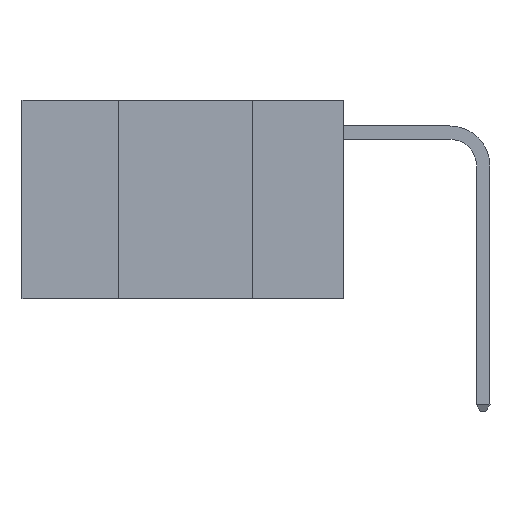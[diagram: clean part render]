
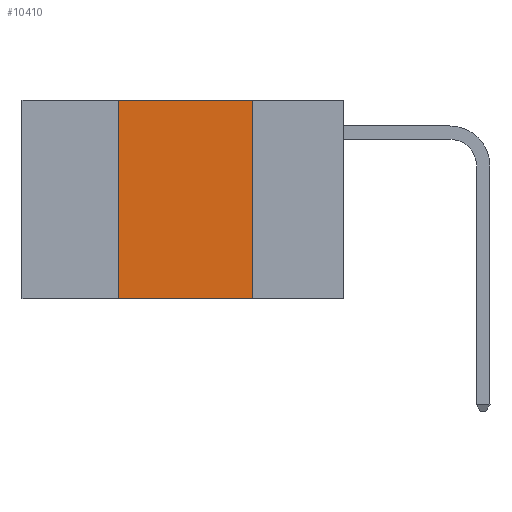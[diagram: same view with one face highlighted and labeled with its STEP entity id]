
A CAD part, left-side view. The second image highlights one B-rep face of the part: STEP entity #10410.
In plain terms, the highlighted planar face has unit normal (-1, 0, 0).
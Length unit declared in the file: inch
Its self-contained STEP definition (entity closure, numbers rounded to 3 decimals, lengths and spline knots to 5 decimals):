
#148 = PLANE ( 'NONE',  #8268 ) ;
#742 = CARTESIAN_POINT ( 'NONE',  ( 0., 0.6, -0.37 ) ) ;
#883 = EDGE_LOOP ( 'NONE', ( #10548, #9997, #11428, #1751 ) ) ;
#1121 = VERTEX_POINT ( 'NONE', #14163 ) ;
#1314 = DIRECTION ( 'NONE',  ( 0., 0., -1. ) ) ;
#1743 = LINE ( 'NONE', #13367, #4738 ) ;
#1751 = ORIENTED_EDGE ( 'NONE', *, *, #13897, .T. ) ;
#2292 = CARTESIAN_POINT ( 'NONE',  ( 0., 0.17, 0. ) ) ;
#2367 = DIRECTION ( 'NONE',  ( 0., 0., -1. ) ) ;
#2444 = VECTOR ( 'NONE', #2367, 39.37008 ) ;
#2475 = LINE ( 'NONE', #2292, #2444 ) ;
#2565 = EDGE_CURVE ( 'NONE', #1121, #4885, #2475, .T. ) ;
#3394 = EDGE_CURVE ( 'NONE', #5952, #9579, #13083, .T. ) ;
#4494 = LINE ( 'NONE', #742, #10064 ) ;
#4738 = VECTOR ( 'NONE', #6932, 39.37008 ) ;
#4885 = VERTEX_POINT ( 'NONE', #10338 ) ;
#5952 = VERTEX_POINT ( 'NONE', #7999 ) ;
#6932 = DIRECTION ( 'NONE',  ( 0., -1., 0. ) ) ;
#7334 = FACE_OUTER_BOUND ( 'NONE', #883, .T. ) ;
#7999 = CARTESIAN_POINT ( 'NONE',  ( 0., 0.42, -0.37 ) ) ;
#8111 = DIRECTION ( 'NONE',  ( 1., 0., 0. ) ) ;
#8268 = AXIS2_PLACEMENT_3D ( 'NONE', #10207, #8111, #1314 ) ;
#9579 = VERTEX_POINT ( 'NONE', #12835 ) ;
#9997 = ORIENTED_EDGE ( 'NONE', *, *, #12169, .F. ) ;
#10064 = VECTOR ( 'NONE', #11868, 39.37008 ) ;
#10207 = CARTESIAN_POINT ( 'NONE',  ( 0., 0.6, 0. ) ) ;
#10338 = CARTESIAN_POINT ( 'NONE',  ( 0., 0.17, -0.37 ) ) ;
#10410 = ADVANCED_FACE ( 'NONE', ( #7334 ), #148, .F. ) ;
#10548 = ORIENTED_EDGE ( 'NONE', *, *, #2565, .F. ) ;
#11127 = DIRECTION ( 'NONE',  ( 0., 0., 1. ) ) ;
#11274 = CARTESIAN_POINT ( 'NONE',  ( 0., 0.42, 0. ) ) ;
#11428 = ORIENTED_EDGE ( 'NONE', *, *, #3394, .F. ) ;
#11868 = DIRECTION ( 'NONE',  ( 0., -1., 0. ) ) ;
#12169 = EDGE_CURVE ( 'NONE', #9579, #1121, #1743, .T. ) ;
#12835 = CARTESIAN_POINT ( 'NONE',  ( 0., 0.42, 0. ) ) ;
#13067 = VECTOR ( 'NONE', #11127, 39.37008 ) ;
#13083 = LINE ( 'NONE', #11274, #13067 ) ;
#13367 = CARTESIAN_POINT ( 'NONE',  ( 0., 0.6, 0. ) ) ;
#13897 = EDGE_CURVE ( 'NONE', #5952, #4885, #4494, .T. ) ;
#14163 = CARTESIAN_POINT ( 'NONE',  ( 0., 0.17, 0. ) ) ;
